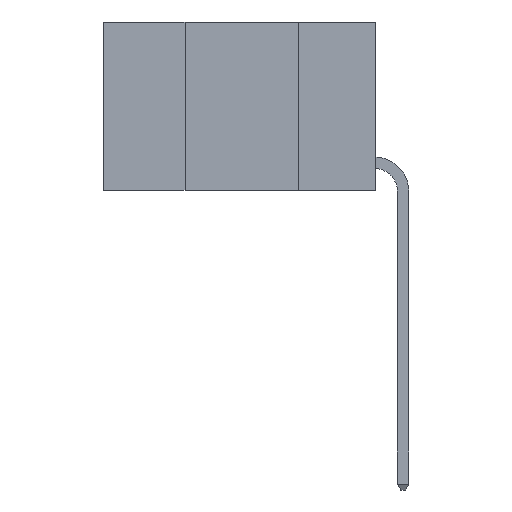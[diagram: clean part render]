
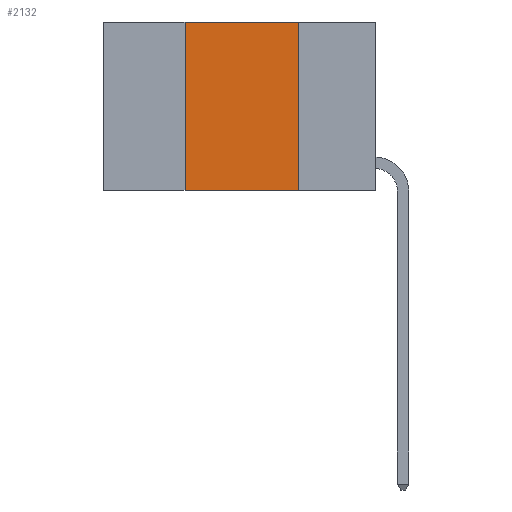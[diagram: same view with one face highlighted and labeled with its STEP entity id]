
A CAD part, left-side view. The second image highlights one B-rep face of the part: STEP entity #2132.
In plain terms, the highlighted planar face has unit normal (-1, 0, 0).
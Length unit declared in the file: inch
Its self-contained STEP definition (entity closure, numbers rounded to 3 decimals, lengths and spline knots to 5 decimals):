
#442 = ORIENTED_EDGE ( 'NONE', *, *, #8253, .T. ) ;
#603 = VERTEX_POINT ( 'NONE', #1152 ) ;
#957 = VECTOR ( 'NONE', #4019, 39.37008 ) ;
#1150 = LINE ( 'NONE', #4194, #957 ) ;
#1152 = CARTESIAN_POINT ( 'NONE',  ( 0., 0.17, 0. ) ) ;
#1241 = VERTEX_POINT ( 'NONE', #8194 ) ;
#1471 = CARTESIAN_POINT ( 'NONE',  ( 0., 0.17, -0.37 ) ) ;
#2007 = ORIENTED_EDGE ( 'NONE', *, *, #4930, .F. ) ;
#2132 = ADVANCED_FACE ( 'NONE', ( #7255 ), #4902, .F. ) ;
#2302 = CARTESIAN_POINT ( 'NONE',  ( 0., 0.42, -0.37 ) ) ;
#2306 = ORIENTED_EDGE ( 'NONE', *, *, #6212, .F. ) ;
#2817 = VERTEX_POINT ( 'NONE', #2302 ) ;
#2886 = VERTEX_POINT ( 'NONE', #1471 ) ;
#2967 = ORIENTED_EDGE ( 'NONE', *, *, #3936, .F. ) ;
#3631 = CARTESIAN_POINT ( 'NONE',  ( 0., 0.6, -0.37 ) ) ;
#3824 = AXIS2_PLACEMENT_3D ( 'NONE', #4729, #4660, #4581 ) ;
#3936 = EDGE_CURVE ( 'NONE', #2817, #1241, #5737, .T. ) ;
#4019 = DIRECTION ( 'NONE',  ( 0., 0., -1. ) ) ;
#4194 = CARTESIAN_POINT ( 'NONE',  ( 0., 0.17, 0. ) ) ;
#4510 = VECTOR ( 'NONE', #8251, 39.37008 ) ;
#4581 = DIRECTION ( 'NONE',  ( 0., 0., -1. ) ) ;
#4660 = DIRECTION ( 'NONE',  ( 1., 0., 0. ) ) ;
#4729 = CARTESIAN_POINT ( 'NONE',  ( 0., 0.6, 0. ) ) ;
#4902 = PLANE ( 'NONE',  #3824 ) ;
#4930 = EDGE_CURVE ( 'NONE', #603, #2886, #1150, .T. ) ;
#5510 = DIRECTION ( 'NONE',  ( 0., -1., 0. ) ) ;
#5686 = CARTESIAN_POINT ( 'NONE',  ( 0., 0.6, 0. ) ) ;
#5737 = LINE ( 'NONE', #8247, #4510 ) ;
#6127 = VECTOR ( 'NONE', #5510, 39.37008 ) ;
#6212 = EDGE_CURVE ( 'NONE', #1241, #603, #8680, .T. ) ;
#7255 = FACE_OUTER_BOUND ( 'NONE', #8147, .T. ) ;
#7639 = DIRECTION ( 'NONE',  ( 0., -1., 0. ) ) ;
#8147 = EDGE_LOOP ( 'NONE', ( #2007, #2306, #2967, #442 ) ) ;
#8194 = CARTESIAN_POINT ( 'NONE',  ( 0., 0.42, 0. ) ) ;
#8233 = VECTOR ( 'NONE', #7639, 39.37008 ) ;
#8247 = CARTESIAN_POINT ( 'NONE',  ( 0., 0.42, 0. ) ) ;
#8251 = DIRECTION ( 'NONE',  ( 0., 0., 1. ) ) ;
#8253 = EDGE_CURVE ( 'NONE', #2817, #2886, #8422, .T. ) ;
#8422 = LINE ( 'NONE', #3631, #8233 ) ;
#8680 = LINE ( 'NONE', #5686, #6127 ) ;
